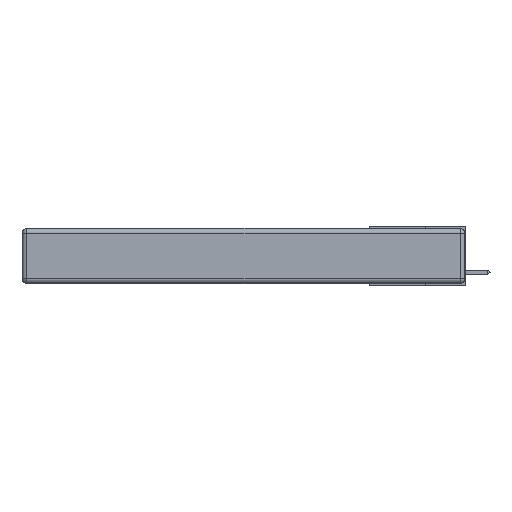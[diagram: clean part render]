
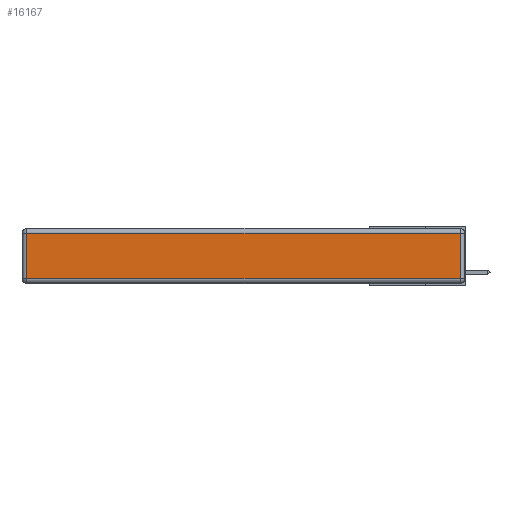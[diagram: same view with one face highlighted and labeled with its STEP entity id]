
A CAD part, left-side view. The second image highlights one B-rep face of the part: STEP entity #16167.
In plain terms, the highlighted planar face has unit normal (-1, 0, 0).
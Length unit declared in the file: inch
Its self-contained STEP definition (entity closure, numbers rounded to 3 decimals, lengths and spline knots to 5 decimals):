
#1145 = CARTESIAN_POINT ( 'NONE',  ( 0., 2.75, -0.03 ) ) ;
#1542 = VECTOR ( 'NONE', #4529, 39.37008 ) ;
#2109 = EDGE_CURVE ( 'NONE', #15126, #19998, #3923, .T. ) ;
#3167 = CARTESIAN_POINT ( 'NONE',  ( 0., 0.03, -0.343 ) ) ;
#3923 = LINE ( 'NONE', #17733, #21104 ) ;
#4529 = DIRECTION ( 'NONE',  ( 0., 0., -1. ) ) ;
#4758 = VECTOR ( 'NONE', #21997, 39.37008 ) ;
#5471 = LINE ( 'NONE', #3167, #20470 ) ;
#5602 = ORIENTED_EDGE ( 'NONE', *, *, #2109, .T. ) ;
#5927 = ORIENTED_EDGE ( 'NONE', *, *, #19653, .T. ) ;
#5947 = PLANE ( 'NONE',  #9691 ) ;
#5963 = EDGE_LOOP ( 'NONE', ( #5602, #10312, #13450, #5927 ) ) ;
#9691 = AXIS2_PLACEMENT_3D ( 'NONE', #27042, #12891, #15278 ) ;
#10132 = DIRECTION ( 'NONE',  ( 0., 0., 1. ) ) ;
#10312 = ORIENTED_EDGE ( 'NONE', *, *, #21199, .T. ) ;
#12135 = VERTEX_POINT ( 'NONE', #17223 ) ;
#12891 = DIRECTION ( 'NONE',  ( -1., 0., 0. ) ) ;
#13450 = ORIENTED_EDGE ( 'NONE', *, *, #29965, .T. ) ;
#14279 = LINE ( 'NONE', #1145, #4758 ) ;
#15126 = VERTEX_POINT ( 'NONE', #23124 ) ;
#15266 = DIRECTION ( 'NONE',  ( 0., -1., 0. ) ) ;
#15278 = DIRECTION ( 'NONE',  ( 0., 0., 1. ) ) ;
#16167 = ADVANCED_FACE ( 'NONE', ( #17494 ), #5947, .T. ) ;
#16590 = LINE ( 'NONE', #22313, #1542 ) ;
#17223 = CARTESIAN_POINT ( 'NONE',  ( 0., 2.72, -0.03 ) ) ;
#17494 = FACE_OUTER_BOUND ( 'NONE', #5963, .T. ) ;
#17733 = CARTESIAN_POINT ( 'NONE',  ( 0., 0., -0.313 ) ) ;
#19653 = EDGE_CURVE ( 'NONE', #12135, #15126, #16590, .T. ) ;
#19986 = CARTESIAN_POINT ( 'NONE',  ( 0., 0.03, -0.313 ) ) ;
#19998 = VERTEX_POINT ( 'NONE', #19986 ) ;
#20470 = VECTOR ( 'NONE', #10132, 39.37008 ) ;
#21009 = VERTEX_POINT ( 'NONE', #23736 ) ;
#21104 = VECTOR ( 'NONE', #15266, 39.37008 ) ;
#21199 = EDGE_CURVE ( 'NONE', #19998, #21009, #5471, .T. ) ;
#21997 = DIRECTION ( 'NONE',  ( 0., 1., 0. ) ) ;
#22313 = CARTESIAN_POINT ( 'NONE',  ( 0., 2.72, -0.343 ) ) ;
#23124 = CARTESIAN_POINT ( 'NONE',  ( 0., 2.72, -0.313 ) ) ;
#23736 = CARTESIAN_POINT ( 'NONE',  ( 0., 0.03, -0.03 ) ) ;
#27042 = CARTESIAN_POINT ( 'NONE',  ( 0., 0., -0.343 ) ) ;
#29965 = EDGE_CURVE ( 'NONE', #21009, #12135, #14279, .T. ) ;
